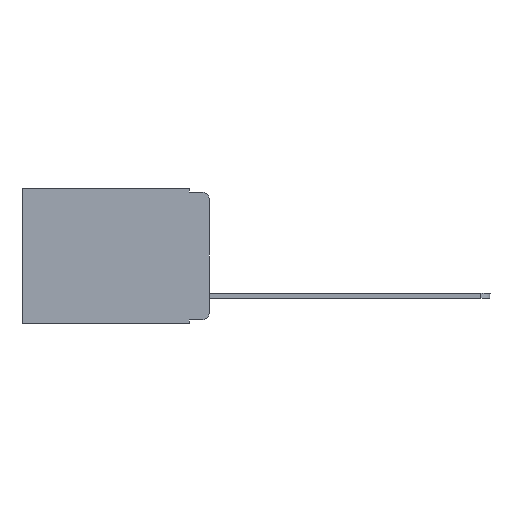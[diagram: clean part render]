
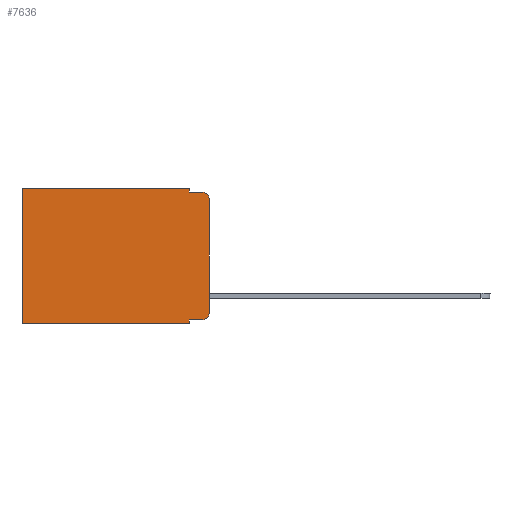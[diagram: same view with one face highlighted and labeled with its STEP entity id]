
A CAD part, left-side view. The second image highlights one B-rep face of the part: STEP entity #7636.
In plain terms, the highlighted planar face has unit normal (-1, 0, 0).
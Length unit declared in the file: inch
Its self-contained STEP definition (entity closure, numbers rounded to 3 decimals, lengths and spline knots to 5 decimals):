
#91 = ORIENTED_EDGE ( 'NONE', *, *, #7768, .F. ) ;
#98 = CARTESIAN_POINT ( 'NONE',  ( 0.298, 0.051, 0. ) ) ;
#108 = LINE ( 'NONE', #3211, #3340 ) ;
#379 = VERTEX_POINT ( 'NONE', #8973 ) ;
#780 = CARTESIAN_POINT ( 'NONE',  ( 0.298, 0., 0. ) ) ;
#807 = VECTOR ( 'NONE', #8086, 39.37008 ) ;
#816 = DIRECTION ( 'NONE',  ( -1., 0., 0. ) ) ;
#910 = EDGE_CURVE ( 'NONE', #6262, #6790, #4000, .T. ) ;
#926 = EDGE_CURVE ( 'NONE', #8628, #379, #8478, .T. ) ;
#1028 = CARTESIAN_POINT ( 'NONE',  ( 0.298, 0., 0. ) ) ;
#1210 = LINE ( 'NONE', #7237, #9066 ) ;
#1255 = LINE ( 'NONE', #1305, #4581 ) ;
#1305 = CARTESIAN_POINT ( 'NONE',  ( 0.298, 0.051, 0. ) ) ;
#1337 = CIRCLE ( 'NONE', #2335, 0.02 ) ;
#1442 = FACE_OUTER_BOUND ( 'NONE', #3962, .T. ) ;
#1505 = ORIENTED_EDGE ( 'NONE', *, *, #6023, .F. ) ;
#1676 = VECTOR ( 'NONE', #1678, 39.37008 ) ;
#1678 = DIRECTION ( 'NONE',  ( 0., 0., -1. ) ) ;
#1938 = EDGE_CURVE ( 'NONE', #7952, #3092, #1210, .T. ) ;
#1988 = EDGE_CURVE ( 'NONE', #3092, #7036, #2698, .T. ) ;
#2335 = AXIS2_PLACEMENT_3D ( 'NONE', #8539, #816, #5474 ) ;
#2495 = ORIENTED_EDGE ( 'NONE', *, *, #926, .T. ) ;
#2519 = CARTESIAN_POINT ( 'NONE',  ( 0.298, 0.473, -0.343 ) ) ;
#2698 = LINE ( 'NONE', #5021, #807 ) ;
#2931 = ORIENTED_EDGE ( 'NONE', *, *, #5001, .F. ) ;
#2932 = DIRECTION ( 'NONE',  ( 0., 0., -1. ) ) ;
#3092 = VERTEX_POINT ( 'NONE', #3378 ) ;
#3211 = CARTESIAN_POINT ( 'NONE',  ( 0.298, 0., -0.343 ) ) ;
#3340 = VECTOR ( 'NONE', #8549, 39.37008 ) ;
#3378 = CARTESIAN_POINT ( 'NONE',  ( 0.298, 0.473, 0. ) ) ;
#3805 = CARTESIAN_POINT ( 'NONE',  ( 0.298, 0.051, -0.333 ) ) ;
#3962 = EDGE_LOOP ( 'NONE', ( #91, #7646, #4832, #1505, #6115, #7071, #9284, #2931, #2495, #8201 ) ) ;
#4000 = LINE ( 'NONE', #7815, #8055 ) ;
#4005 = DIRECTION ( 'NONE',  ( -1., 0., 0. ) ) ;
#4581 = VECTOR ( 'NONE', #8956, 39.37008 ) ;
#4639 = CARTESIAN_POINT ( 'NONE',  ( 0.298, 0., -0.313 ) ) ;
#4832 = ORIENTED_EDGE ( 'NONE', *, *, #910, .F. ) ;
#5001 = EDGE_CURVE ( 'NONE', #8628, #6331, #1255, .T. ) ;
#5021 = CARTESIAN_POINT ( 'NONE',  ( 0.298, 0.473, 0. ) ) ;
#5474 = DIRECTION ( 'NONE',  ( 0., 0., -1. ) ) ;
#5589 = DIRECTION ( 'NONE',  ( 0., 0., -1. ) ) ;
#5919 = AXIS2_PLACEMENT_3D ( 'NONE', #8688, #4005, #7869 ) ;
#6010 = EDGE_CURVE ( 'NONE', #9269, #6790, #1337, .T. ) ;
#6023 = EDGE_CURVE ( 'NONE', #7952, #6262, #6984, .T. ) ;
#6062 = CARTESIAN_POINT ( 'NONE',  ( 0.298, 0.02, -0.01 ) ) ;
#6115 = ORIENTED_EDGE ( 'NONE', *, *, #1938, .T. ) ;
#6262 = VERTEX_POINT ( 'NONE', #8082 ) ;
#6314 = CARTESIAN_POINT ( 'NONE',  ( 0.298, 0.051, -0.333 ) ) ;
#6331 = VERTEX_POINT ( 'NONE', #9072 ) ;
#6790 = VERTEX_POINT ( 'NONE', #6062 ) ;
#6874 = DIRECTION ( 'NONE',  ( 0., -1., 0. ) ) ;
#6984 = LINE ( 'NONE', #98, #1676 ) ;
#7036 = VERTEX_POINT ( 'NONE', #2519 ) ;
#7071 = ORIENTED_EDGE ( 'NONE', *, *, #1988, .T. ) ;
#7237 = CARTESIAN_POINT ( 'NONE',  ( 0.298, 0., 0. ) ) ;
#7427 = VECTOR ( 'NONE', #5589, 39.37008 ) ;
#7538 = VERTEX_POINT ( 'NONE', #4639 ) ;
#7636 = ADVANCED_FACE ( 'NONE', ( #1442 ), #10002, .F. ) ;
#7646 = ORIENTED_EDGE ( 'NONE', *, *, #6010, .T. ) ;
#7768 = EDGE_CURVE ( 'NONE', #9269, #7538, #7950, .T. ) ;
#7815 = CARTESIAN_POINT ( 'NONE',  ( 0.298, 0.051, -0.01 ) ) ;
#7869 = DIRECTION ( 'NONE',  ( 0., 0., -1. ) ) ;
#7950 = LINE ( 'NONE', #1028, #7427 ) ;
#7952 = VERTEX_POINT ( 'NONE', #8870 ) ;
#7980 = DIRECTION ( 'NONE',  ( 0., 1., 0. ) ) ;
#8055 = VECTOR ( 'NONE', #6874, 39.37008 ) ;
#8082 = CARTESIAN_POINT ( 'NONE',  ( 0.298, 0.051, -0.01 ) ) ;
#8086 = DIRECTION ( 'NONE',  ( 0., 0., -1. ) ) ;
#8201 = ORIENTED_EDGE ( 'NONE', *, *, #9751, .T. ) ;
#8478 = LINE ( 'NONE', #3805, #9059 ) ;
#8507 = DIRECTION ( 'NONE',  ( 1., 0., 0. ) ) ;
#8539 = CARTESIAN_POINT ( 'NONE',  ( 0.298, 0.02, -0.03 ) ) ;
#8549 = DIRECTION ( 'NONE',  ( 0., 1., 0. ) ) ;
#8628 = VERTEX_POINT ( 'NONE', #6314 ) ;
#8688 = CARTESIAN_POINT ( 'NONE',  ( 0.298, 0.02, -0.313 ) ) ;
#8870 = CARTESIAN_POINT ( 'NONE',  ( 0.298, 0.051, 0. ) ) ;
#8956 = DIRECTION ( 'NONE',  ( 0., 0., -1. ) ) ;
#8973 = CARTESIAN_POINT ( 'NONE',  ( 0.298, 0.02, -0.333 ) ) ;
#9059 = VECTOR ( 'NONE', #9367, 39.37008 ) ;
#9066 = VECTOR ( 'NONE', #7980, 39.37008 ) ;
#9072 = CARTESIAN_POINT ( 'NONE',  ( 0.298, 0.051, -0.343 ) ) ;
#9269 = VERTEX_POINT ( 'NONE', #9993 ) ;
#9284 = ORIENTED_EDGE ( 'NONE', *, *, #9325, .F. ) ;
#9325 = EDGE_CURVE ( 'NONE', #6331, #7036, #108, .T. ) ;
#9367 = DIRECTION ( 'NONE',  ( 0., -1., 0. ) ) ;
#9484 = CIRCLE ( 'NONE', #5919, 0.02 ) ;
#9751 = EDGE_CURVE ( 'NONE', #379, #7538, #9484, .T. ) ;
#9767 = AXIS2_PLACEMENT_3D ( 'NONE', #780, #8507, #2932 ) ;
#9993 = CARTESIAN_POINT ( 'NONE',  ( 0.298, 0., -0.03 ) ) ;
#10002 = PLANE ( 'NONE',  #9767 ) ;
